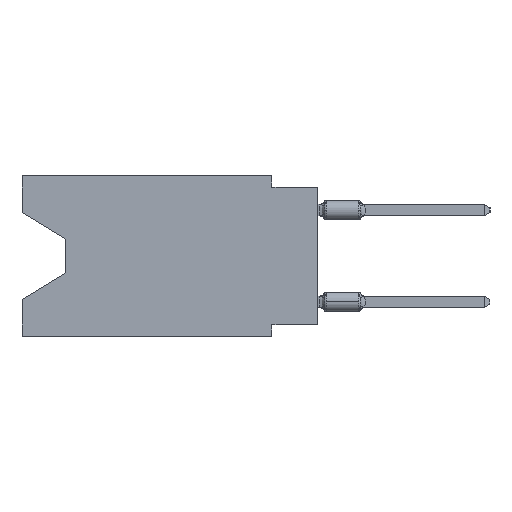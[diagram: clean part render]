
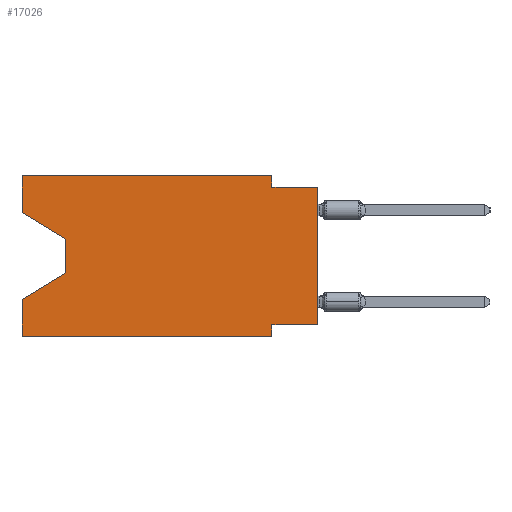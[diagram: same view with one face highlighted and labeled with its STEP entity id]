
A CAD part, left-side view. The second image highlights one B-rep face of the part: STEP entity #17026.
In plain terms, the highlighted planar face has unit normal (-1, 0, 0).
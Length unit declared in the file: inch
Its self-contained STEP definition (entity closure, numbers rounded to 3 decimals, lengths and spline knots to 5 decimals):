
#689 = DIRECTION ( 'NONE',  ( 0., -1., 0. ) ) ;
#1155 = CARTESIAN_POINT ( 'NONE',  ( 0., 0.55, -0.212 ) ) ;
#1579 = CARTESIAN_POINT ( 'NONE',  ( 0., 0.55, -0.212 ) ) ;
#1782 = EDGE_LOOP ( 'NONE', ( #29424, #35529, #21955, #20814, #17869, #39498, #6482, #19252, #18783, #29793, #1987, #27968 ) ) ;
#1810 = VECTOR ( 'NONE', #689, 39.37008 ) ;
#1942 = EDGE_CURVE ( 'NONE', #34842, #20857, #16245, .T. ) ;
#1987 = ORIENTED_EDGE ( 'NONE', *, *, #1942, .F. ) ;
#2227 = VECTOR ( 'NONE', #45697, 39.37008 ) ;
#2255 = AXIS2_PLACEMENT_3D ( 'NONE', #10895, #43012, #35814 ) ;
#2675 = VERTEX_POINT ( 'NONE', #28468 ) ;
#3160 = EDGE_CURVE ( 'NONE', #12644, #33821, #3315, .T. ) ;
#3315 = LINE ( 'NONE', #6619, #2227 ) ;
#3858 = VERTEX_POINT ( 'NONE', #21114 ) ;
#5037 = VERTEX_POINT ( 'NONE', #5369 ) ;
#5369 = CARTESIAN_POINT ( 'NONE',  ( 0., 0.645, -0.35 ) ) ;
#5532 = LINE ( 'NONE', #18821, #42917 ) ;
#6482 = ORIENTED_EDGE ( 'NONE', *, *, #40446, .F. ) ;
#6619 = CARTESIAN_POINT ( 'NONE',  ( 0., 0., 0. ) ) ;
#7922 = CARTESIAN_POINT ( 'NONE',  ( 0., 0.1, 0. ) ) ;
#9072 = LINE ( 'NONE', #22603, #32408 ) ;
#9289 = DIRECTION ( 'NONE',  ( 0., -1., 0. ) ) ;
#10895 = CARTESIAN_POINT ( 'NONE',  ( 0., 0.645, 0. ) ) ;
#11368 = VERTEX_POINT ( 'NONE', #42663 ) ;
#12406 = VERTEX_POINT ( 'NONE', #40862 ) ;
#12583 = DIRECTION ( 'NONE',  ( 0., 0., -1. ) ) ;
#12644 = VERTEX_POINT ( 'NONE', #28059 ) ;
#12836 = CARTESIAN_POINT ( 'NONE',  ( 0., 0.1, -0.35 ) ) ;
#13527 = EDGE_CURVE ( 'NONE', #29725, #12406, #36063, .T. ) ;
#14599 = FACE_OUTER_BOUND ( 'NONE', #1782, .T. ) ;
#14717 = VECTOR ( 'NONE', #25848, 39.37008 ) ;
#14869 = EDGE_CURVE ( 'NONE', #20857, #11368, #25389, .T. ) ;
#14910 = EDGE_CURVE ( 'NONE', #11368, #33821, #16018, .T. ) ;
#15085 = PLANE ( 'NONE',  #2255 ) ;
#15163 = EDGE_CURVE ( 'NONE', #3858, #22403, #44727, .T. ) ;
#15803 = DIRECTION ( 'NONE',  ( 0., -1., 0. ) ) ;
#16018 = LINE ( 'NONE', #44416, #41515 ) ;
#16116 = CARTESIAN_POINT ( 'NONE',  ( 0., 0.645, -0.08025 ) ) ;
#16245 = LINE ( 'NONE', #41156, #24384 ) ;
#16979 = VECTOR ( 'NONE', #34263, 39.37008 ) ;
#17026 = ADVANCED_FACE ( 'NONE', ( #14599 ), #15085, .F. ) ;
#17869 = ORIENTED_EDGE ( 'NONE', *, *, #23336, .T. ) ;
#18690 = DIRECTION ( 'NONE',  ( 0., 0., 1. ) ) ;
#18783 = ORIENTED_EDGE ( 'NONE', *, *, #14910, .F. ) ;
#18821 = CARTESIAN_POINT ( 'NONE',  ( 0., 0.645, -0.08025 ) ) ;
#19252 = ORIENTED_EDGE ( 'NONE', *, *, #3160, .T. ) ;
#20814 = ORIENTED_EDGE ( 'NONE', *, *, #28162, .F. ) ;
#20857 = VERTEX_POINT ( 'NONE', #35986 ) ;
#21114 = CARTESIAN_POINT ( 'NONE',  ( 0., 0.1, -0.325 ) ) ;
#21955 = ORIENTED_EDGE ( 'NONE', *, *, #13527, .T. ) ;
#22403 = VERTEX_POINT ( 'NONE', #28303 ) ;
#22603 = CARTESIAN_POINT ( 'NONE',  ( 0., 0., -0.325 ) ) ;
#22708 = VERTEX_POINT ( 'NONE', #16116 ) ;
#23336 = EDGE_CURVE ( 'NONE', #5037, #22403, #29097, .T. ) ;
#24384 = VECTOR ( 'NONE', #9289, 39.37008 ) ;
#25161 = VECTOR ( 'NONE', #18690, 39.37008 ) ;
#25389 = LINE ( 'NONE', #7922, #14717 ) ;
#25829 = CARTESIAN_POINT ( 'NONE',  ( 0., 0.645, -0.35 ) ) ;
#25848 = DIRECTION ( 'NONE',  ( 0., 0., -1. ) ) ;
#26159 = CARTESIAN_POINT ( 'NONE',  ( 0., 0.645, 0. ) ) ;
#26380 = CARTESIAN_POINT ( 'NONE',  ( 0., 0.55, -0.138 ) ) ;
#27712 = CARTESIAN_POINT ( 'NONE',  ( 0., 0.645, 0. ) ) ;
#27968 = ORIENTED_EDGE ( 'NONE', *, *, #35463, .F. ) ;
#28059 = CARTESIAN_POINT ( 'NONE',  ( 0., 0., -0.325 ) ) ;
#28162 = EDGE_CURVE ( 'NONE', #5037, #12406, #45359, .T. ) ;
#28303 = CARTESIAN_POINT ( 'NONE',  ( 0., 0.1, -0.35 ) ) ;
#28468 = CARTESIAN_POINT ( 'NONE',  ( 0., 0.55, -0.138 ) ) ;
#29097 = LINE ( 'NONE', #25829, #1810 ) ;
#29424 = ORIENTED_EDGE ( 'NONE', *, *, #34796, .T. ) ;
#29725 = VERTEX_POINT ( 'NONE', #1579 ) ;
#29793 = ORIENTED_EDGE ( 'NONE', *, *, #14869, .F. ) ;
#32408 = VECTOR ( 'NONE', #37457, 39.37008 ) ;
#32866 = LINE ( 'NONE', #26159, #25161 ) ;
#32910 = CARTESIAN_POINT ( 'NONE',  ( 0., 0., -0.025 ) ) ;
#33213 = DIRECTION ( 'NONE',  ( 0., -0.855, -0.519 ) ) ;
#33234 = VECTOR ( 'NONE', #12583, 39.37008 ) ;
#33821 = VERTEX_POINT ( 'NONE', #32910 ) ;
#34263 = DIRECTION ( 'NONE',  ( 0., 0., -1. ) ) ;
#34433 = EDGE_CURVE ( 'NONE', #2675, #29725, #44473, .T. ) ;
#34796 = EDGE_CURVE ( 'NONE', #22708, #2675, #5532, .T. ) ;
#34842 = VERTEX_POINT ( 'NONE', #41339 ) ;
#35463 = EDGE_CURVE ( 'NONE', #22708, #34842, #32866, .T. ) ;
#35529 = ORIENTED_EDGE ( 'NONE', *, *, #34433, .T. ) ;
#35814 = DIRECTION ( 'NONE',  ( 0., 0., -1. ) ) ;
#35986 = CARTESIAN_POINT ( 'NONE',  ( 0., 0.1, 0. ) ) ;
#36063 = LINE ( 'NONE', #1155, #42239 ) ;
#36536 = DIRECTION ( 'NONE',  ( 0., 0.855, -0.519 ) ) ;
#37457 = DIRECTION ( 'NONE',  ( 0., 1., 0. ) ) ;
#38606 = DIRECTION ( 'NONE',  ( 0., 0., 1. ) ) ;
#39498 = ORIENTED_EDGE ( 'NONE', *, *, #15163, .F. ) ;
#40446 = EDGE_CURVE ( 'NONE', #12644, #3858, #9072, .T. ) ;
#40862 = CARTESIAN_POINT ( 'NONE',  ( 0., 0.645, -0.26975 ) ) ;
#41156 = CARTESIAN_POINT ( 'NONE',  ( 0., 0.645, 0. ) ) ;
#41339 = CARTESIAN_POINT ( 'NONE',  ( 0., 0.645, 0. ) ) ;
#41515 = VECTOR ( 'NONE', #15803, 39.37008 ) ;
#42239 = VECTOR ( 'NONE', #36536, 39.37008 ) ;
#42663 = CARTESIAN_POINT ( 'NONE',  ( 0., 0.1, -0.025 ) ) ;
#42917 = VECTOR ( 'NONE', #33213, 39.37008 ) ;
#43012 = DIRECTION ( 'NONE',  ( 1., 0., 0. ) ) ;
#44089 = VECTOR ( 'NONE', #38606, 39.37008 ) ;
#44416 = CARTESIAN_POINT ( 'NONE',  ( 0., 0., -0.025 ) ) ;
#44473 = LINE ( 'NONE', #26380, #33234 ) ;
#44727 = LINE ( 'NONE', #12836, #16979 ) ;
#45359 = LINE ( 'NONE', #27712, #44089 ) ;
#45697 = DIRECTION ( 'NONE',  ( 0., 0., 1. ) ) ;
